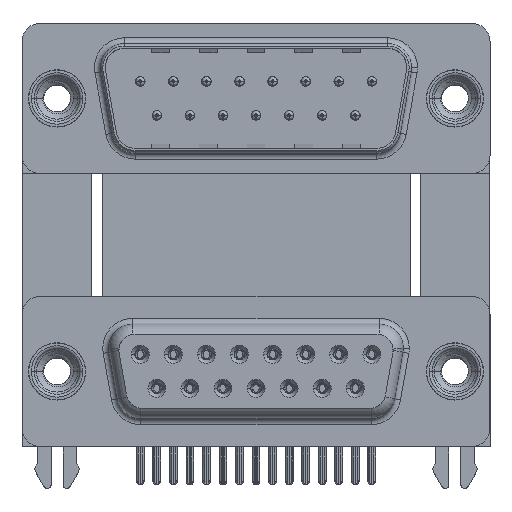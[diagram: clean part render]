
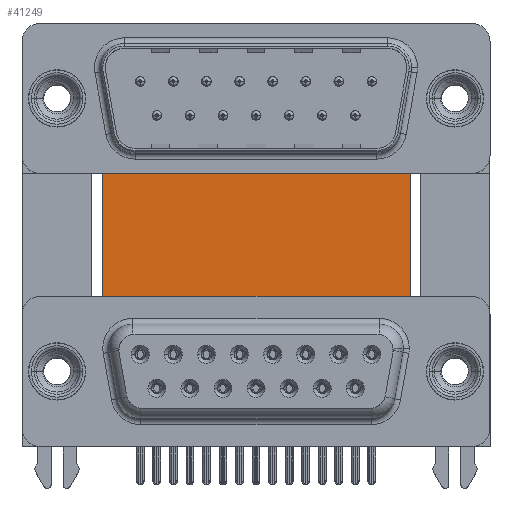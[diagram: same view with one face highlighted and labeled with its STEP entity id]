
A CAD part, top view. The second image highlights one B-rep face of the part: STEP entity #41249.
In plain terms, the highlighted planar face has unit normal (0, 0, 1).
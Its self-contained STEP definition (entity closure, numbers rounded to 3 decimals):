
#705 = CARTESIAN_POINT ( 'NONE',  ( 29.58, 16.585, -12. ) ) ;
#1200 = CARTESIAN_POINT ( 'NONE',  ( 29.58, 16.585, -12. ) ) ;
#3926 = DIRECTION ( 'NONE',  ( 1., 0., 0. ) ) ;
#5244 = ORIENTED_EDGE ( 'NONE', *, *, #33675, .F. ) ;
#12981 = FACE_OUTER_BOUND ( 'NONE', #21134, .T. ) ;
#13735 = VERTEX_POINT ( 'NONE', #705 ) ;
#14817 = VECTOR ( 'NONE', #33203, 1000. ) ;
#15057 = CARTESIAN_POINT ( 'NONE',  ( 3.79, -3.735, -12. ) ) ;
#16436 = VERTEX_POINT ( 'NONE', #20447 ) ;
#17452 = PLANE ( 'NONE',  #39118 ) ;
#18696 = ORIENTED_EDGE ( 'NONE', *, *, #37234, .F. ) ;
#20447 = CARTESIAN_POINT ( 'NONE',  ( 3.79, 16.585, -12. ) ) ;
#21072 = ORIENTED_EDGE ( 'NONE', *, *, #40377, .T. ) ;
#21101 = LINE ( 'NONE', #46101, #37538 ) ;
#21134 = EDGE_LOOP ( 'NONE', ( #45310, #18696, #5244, #21072 ) ) ;
#21151 = VERTEX_POINT ( 'NONE', #33987 ) ;
#21200 = CARTESIAN_POINT ( 'NONE',  ( 29.58, -3.735, -12. ) ) ;
#21840 = CARTESIAN_POINT ( 'NONE',  ( 3.79, 16.585, -12. ) ) ;
#24718 = VERTEX_POINT ( 'NONE', #21200 ) ;
#28283 = DIRECTION ( 'NONE',  ( -1., 0., 0. ) ) ;
#28433 = VECTOR ( 'NONE', #44569, 1000. ) ;
#31834 = DIRECTION ( 'NONE',  ( 0., 0., -1. ) ) ;
#32185 = DIRECTION ( 'NONE',  ( 0., -1., 0. ) ) ;
#33203 = DIRECTION ( 'NONE',  ( 1., 0., 0. ) ) ;
#33660 = LINE ( 'NONE', #15057, #14817 ) ;
#33675 = EDGE_CURVE ( 'NONE', #16436, #13735, #39737, .T. ) ;
#33987 = CARTESIAN_POINT ( 'NONE',  ( 3.79, -3.735, -12. ) ) ;
#37234 = EDGE_CURVE ( 'NONE', #13735, #24718, #43862, .T. ) ;
#37538 = VECTOR ( 'NONE', #32185, 1000. ) ;
#37683 = EDGE_CURVE ( 'NONE', #21151, #24718, #33660, .T. ) ;
#39118 = AXIS2_PLACEMENT_3D ( 'NONE', #42656, #31834, #28283 ) ;
#39737 = LINE ( 'NONE', #21840, #41631 ) ;
#40377 = EDGE_CURVE ( 'NONE', #16436, #21151, #21101, .T. ) ;
#41249 = ADVANCED_FACE ( 'NONE', ( #12981 ), #17452, .F. ) ;
#41631 = VECTOR ( 'NONE', #3926, 1000. ) ;
#42656 = CARTESIAN_POINT ( 'NONE',  ( 3.79, 16.585, -12. ) ) ;
#43862 = LINE ( 'NONE', #1200, #28433 ) ;
#44569 = DIRECTION ( 'NONE',  ( 0., -1., 0. ) ) ;
#45310 = ORIENTED_EDGE ( 'NONE', *, *, #37683, .T. ) ;
#46101 = CARTESIAN_POINT ( 'NONE',  ( 3.79, 16.585, -12. ) ) ;
